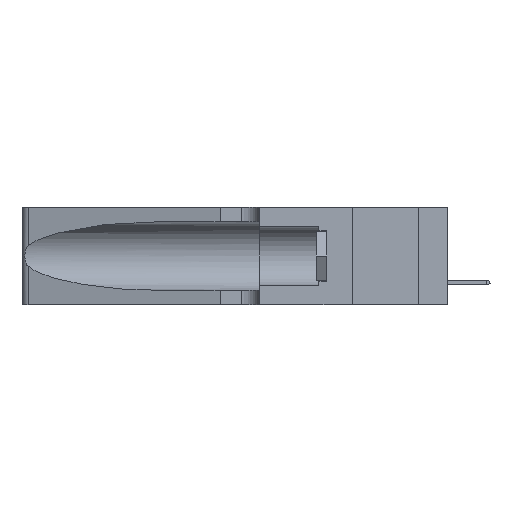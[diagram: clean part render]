
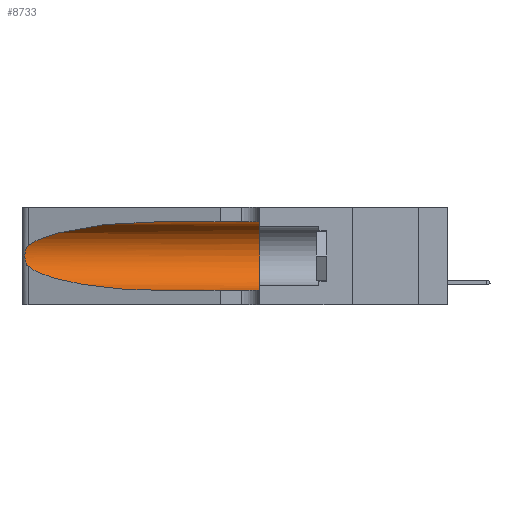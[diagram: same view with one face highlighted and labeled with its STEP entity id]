
A CAD part, left-side view. The second image highlights one B-rep face of the part: STEP entity #8733.
In plain terms, the highlighted cylindrical face has radius 3.308 mm (diameter 6.617 mm), a partial arc.
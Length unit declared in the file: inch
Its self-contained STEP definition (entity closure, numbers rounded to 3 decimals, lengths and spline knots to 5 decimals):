
#51 = ORIENTED_EDGE ( 'NONE', *, *, #18258, .F. ) ;
#501 =( BOUNDED_CURVE ( )  B_SPLINE_CURVE ( 3, ( #1592, #10789, #1282, #29453 ),
 .UNSPECIFIED., .F., .F. ) 
 B_SPLINE_CURVE_WITH_KNOTS ( ( 4, 4 ),
 ( 1.5708, 2.84003 ),
 .UNSPECIFIED. ) 
 CURVE ( )  GEOMETRIC_REPRESENTATION_ITEM ( )  RATIONAL_B_SPLINE_CURVE ( ( 1., 0.87, 0.87, 1. ) ) 
 REPRESENTATION_ITEM ( '' )  );
#1249 = CARTESIAN_POINT ( 'NONE',  ( 0.25487, 1.22718, 0.14631 ) ) ;
#1282 = CARTESIAN_POINT ( 'NONE',  ( 0.2373, 1.15595, 0.28018 ) ) ;
#1516 = VERTEX_POINT ( 'NONE', #10822 ) ;
#1592 = CARTESIAN_POINT ( 'NONE',  ( 0.1305, 0.72297, 0.31525 ) ) ;
#1896 = DIRECTION ( 'NONE',  ( 0., 1., 0. ) ) ;
#1996 = DIRECTION ( 'NONE',  ( 0., 0., 1. ) ) ;
#2518 = ORIENTED_EDGE ( 'NONE', *, *, #14544, .T. ) ;
#3381 = ORIENTED_EDGE ( 'NONE', *, *, #6637, .T. ) ;
#4223 = CARTESIAN_POINT ( 'NONE',  ( 0.1305, 0.35, 0.31525 ) ) ;
#4361 = CARTESIAN_POINT ( 'NONE',  ( 0.26018, 1.23835, 0.19895 ) ) ;
#5480 = CARTESIAN_POINT ( 'NONE',  ( 0.1305, 1.61858, 0.31525 ) ) ;
#5563 =( BOUNDED_CURVE ( )  B_SPLINE_CURVE ( 3, ( #1249, #19829, #22690, #11116 ),
 .UNSPECIFIED., .F., .F. ) 
 B_SPLINE_CURVE_WITH_KNOTS ( ( 4, 4 ),
 ( 3.44316, 4.71239 ),
 .UNSPECIFIED. ) 
 CURVE ( )  GEOMETRIC_REPRESENTATION_ITEM ( )  RATIONAL_B_SPLINE_CURVE ( ( 1., 0.87, 0.87, 1. ) ) 
 REPRESENTATION_ITEM ( '' )  );
#5665 = EDGE_CURVE ( 'NONE', #22204, #27921, #501, .T. ) ;
#5820 = VERTEX_POINT ( 'NONE', #24044 ) ;
#6364 = VECTOR ( 'NONE', #20706, 39.37008 ) ;
#6382 = CARTESIAN_POINT ( 'NONE',  ( 0.1305, 0.35, 0.185 ) ) ;
#6601 = VERTEX_POINT ( 'NONE', #4223 ) ;
#6637 = EDGE_CURVE ( 'NONE', #5820, #12675, #5563, .T. ) ;
#6726 = CARTESIAN_POINT ( 'NONE',  ( 0.25639, 1.23186, 0.15144 ) ) ;
#8268 = CARTESIAN_POINT ( 'NONE',  ( 0.25639, 1.23184, 0.21858 ) ) ;
#8733 = ADVANCED_FACE ( 'NONE', ( #24865 ), #17259, .F. ) ;
#8767 = CARTESIAN_POINT ( 'NONE',  ( 0.1305, 0.72297, 0.05475 ) ) ;
#9458 = ORIENTED_EDGE ( 'NONE', *, *, #5665, .T. ) ;
#9670 = B_SPLINE_CURVE_WITH_KNOTS ( 'NONE', 3,
 ( #21134, #22940, #8268, #25487, #23190, #4361, #27557, #22910, #27651, #11542, #13925, #6726, #27941, #29920 ),
 .UNSPECIFIED., .F., .F.,
 ( 4, 2, 2, 2, 2, 2, 4 ),
 ( 0., 0.00027, 0.00053, 0.00107, 0.0016, 0.00187, 0.00214 ),
 .UNSPECIFIED. ) ;
#10789 = CARTESIAN_POINT ( 'NONE',  ( 0.18966, 0.96281, 0.31525 ) ) ;
#10822 = CARTESIAN_POINT ( 'NONE',  ( 0.1305, 0.35, 0.05475 ) ) ;
#10869 = VECTOR ( 'NONE', #28773, 39.37008 ) ;
#11116 = CARTESIAN_POINT ( 'NONE',  ( 0.1305, 0.72297, 0.05475 ) ) ;
#11542 = CARTESIAN_POINT ( 'NONE',  ( 0.25856, 1.23593, 0.16098 ) ) ;
#12270 = DIRECTION ( 'NONE',  ( 0., 0., -1. ) ) ;
#12675 = VERTEX_POINT ( 'NONE', #8767 ) ;
#13660 = EDGE_CURVE ( 'NONE', #12675, #1516, #26036, .T. ) ;
#13925 = CARTESIAN_POINT ( 'NONE',  ( 0.25789, 1.23486, 0.15765 ) ) ;
#14147 = EDGE_LOOP ( 'NONE', ( #9458, #2518, #3381, #20626, #51, #22228 ) ) ;
#14544 = EDGE_CURVE ( 'NONE', #27921, #5820, #9670, .T. ) ;
#14741 = DIRECTION ( 'NONE',  ( 0., -1., 0. ) ) ;
#17259 = CYLINDRICAL_SURFACE ( 'NONE', #17457, 0.13025 ) ;
#17457 = AXIS2_PLACEMENT_3D ( 'NONE', #26423, #14741, #12270 ) ;
#18258 = EDGE_CURVE ( 'NONE', #6601, #1516, #20470, .T. ) ;
#19829 = CARTESIAN_POINT ( 'NONE',  ( 0.2373, 1.15595, 0.08982 ) ) ;
#20470 = CIRCLE ( 'NONE', #26140, 0.13025 ) ;
#20626 = ORIENTED_EDGE ( 'NONE', *, *, #13660, .T. ) ;
#20706 = DIRECTION ( 'NONE',  ( 0., -1., 0. ) ) ;
#20710 = LINE ( 'NONE', #5480, #10869 ) ;
#20886 = EDGE_CURVE ( 'NONE', #22204, #6601, #20710, .T. ) ;
#21134 = CARTESIAN_POINT ( 'NONE',  ( 0.25487, 1.22718, 0.22369 ) ) ;
#22204 = VERTEX_POINT ( 'NONE', #22869 ) ;
#22228 = ORIENTED_EDGE ( 'NONE', *, *, #20886, .F. ) ;
#22690 = CARTESIAN_POINT ( 'NONE',  ( 0.18966, 0.96281, 0.05475 ) ) ;
#22869 = CARTESIAN_POINT ( 'NONE',  ( 0.1305, 0.72297, 0.31525 ) ) ;
#22910 = CARTESIAN_POINT ( 'NONE',  ( 0.26075, 1.23896, 0.178 ) ) ;
#22940 = CARTESIAN_POINT ( 'NONE',  ( 0.25555, 1.22994, 0.2215 ) ) ;
#23190 = CARTESIAN_POINT ( 'NONE',  ( 0.25854, 1.2359, 0.20912 ) ) ;
#24044 = CARTESIAN_POINT ( 'NONE',  ( 0.25487, 1.22718, 0.14631 ) ) ;
#24865 = FACE_OUTER_BOUND ( 'NONE', #14147, .T. ) ;
#25487 = CARTESIAN_POINT ( 'NONE',  ( 0.25787, 1.23484, 0.2124 ) ) ;
#26036 = LINE ( 'NONE', #26536, #6364 ) ;
#26140 = AXIS2_PLACEMENT_3D ( 'NONE', #6382, #1896, #1996 ) ;
#26423 = CARTESIAN_POINT ( 'NONE',  ( 0.1305, 1.61858, 0.185 ) ) ;
#26536 = CARTESIAN_POINT ( 'NONE',  ( 0.1305, 1.61858, 0.05475 ) ) ;
#27557 = CARTESIAN_POINT ( 'NONE',  ( 0.26075, 1.23896, 0.19203 ) ) ;
#27651 = CARTESIAN_POINT ( 'NONE',  ( 0.26017, 1.23833, 0.17102 ) ) ;
#27921 = VERTEX_POINT ( 'NONE', #29807 ) ;
#27941 = CARTESIAN_POINT ( 'NONE',  ( 0.25555, 1.22993, 0.14849 ) ) ;
#28773 = DIRECTION ( 'NONE',  ( 0., -1., 0. ) ) ;
#29453 = CARTESIAN_POINT ( 'NONE',  ( 0.25487, 1.22718, 0.22369 ) ) ;
#29807 = CARTESIAN_POINT ( 'NONE',  ( 0.25487, 1.22718, 0.22369 ) ) ;
#29920 = CARTESIAN_POINT ( 'NONE',  ( 0.25487, 1.22718, 0.14631 ) ) ;
